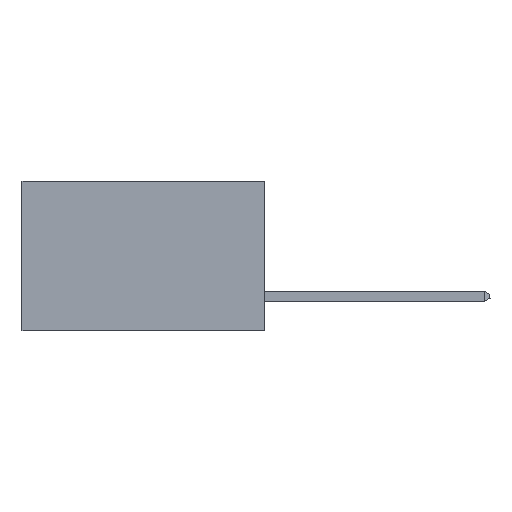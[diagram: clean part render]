
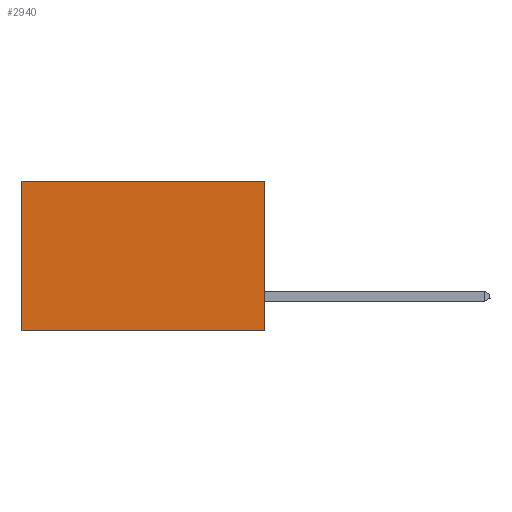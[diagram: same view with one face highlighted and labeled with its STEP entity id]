
A CAD part, left-side view. The second image highlights one B-rep face of the part: STEP entity #2940.
In plain terms, the highlighted planar face has unit normal (-1, 0, 0).
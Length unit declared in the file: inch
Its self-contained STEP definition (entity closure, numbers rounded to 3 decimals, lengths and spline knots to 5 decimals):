
#110 = VERTEX_POINT ( 'NONE', #6450 ) ;
#340 = DIRECTION ( 'NONE',  ( 0., 0., -1. ) ) ;
#413 = CARTESIAN_POINT ( 'NONE',  ( 0.298, 0., -0.37 ) ) ;
#958 = EDGE_CURVE ( 'NONE', #110, #6330, #5982, .T. ) ;
#1073 = EDGE_CURVE ( 'NONE', #6102, #6330, #7921, .T. ) ;
#1095 = EDGE_CURVE ( 'NONE', #4575, #6102, #7491, .T. ) ;
#1909 = CARTESIAN_POINT ( 'NONE',  ( 0.298, 0.6, 0. ) ) ;
#2111 = CARTESIAN_POINT ( 'NONE',  ( 0.298, 0., 0. ) ) ;
#2940 = ADVANCED_FACE ( 'NONE', ( #4148 ), #3633, .F. ) ;
#3633 = PLANE ( 'NONE',  #3737 ) ;
#3737 = AXIS2_PLACEMENT_3D ( 'NONE', #6610, #7228, #5591 ) ;
#3866 = CARTESIAN_POINT ( 'NONE',  ( 0.298, 0., -0.37 ) ) ;
#4030 = LINE ( 'NONE', #4324, #7432 ) ;
#4148 = FACE_OUTER_BOUND ( 'NONE', #8234, .T. ) ;
#4186 = VECTOR ( 'NONE', #8413, 39.37008 ) ;
#4272 = EDGE_CURVE ( 'NONE', #4575, #110, #4030, .T. ) ;
#4324 = CARTESIAN_POINT ( 'NONE',  ( 0.298, 0., 0. ) ) ;
#4575 = VERTEX_POINT ( 'NONE', #2111 ) ;
#5475 = VECTOR ( 'NONE', #340, 39.37008 ) ;
#5591 = DIRECTION ( 'NONE',  ( 0., 0., -1. ) ) ;
#5982 = LINE ( 'NONE', #1909, #4186 ) ;
#6102 = VERTEX_POINT ( 'NONE', #413 ) ;
#6123 = DIRECTION ( 'NONE',  ( 0., 1., 0. ) ) ;
#6330 = VERTEX_POINT ( 'NONE', #8139 ) ;
#6376 = ORIENTED_EDGE ( 'NONE', *, *, #1095, .F. ) ;
#6450 = CARTESIAN_POINT ( 'NONE',  ( 0.298, 0.6, 0. ) ) ;
#6549 = ORIENTED_EDGE ( 'NONE', *, *, #1073, .F. ) ;
#6610 = CARTESIAN_POINT ( 'NONE',  ( 0.298, 0., 0. ) ) ;
#6829 = ORIENTED_EDGE ( 'NONE', *, *, #958, .T. ) ;
#7228 = DIRECTION ( 'NONE',  ( 1., 0., 0. ) ) ;
#7432 = VECTOR ( 'NONE', #9420, 39.37008 ) ;
#7436 = ORIENTED_EDGE ( 'NONE', *, *, #4272, .T. ) ;
#7491 = LINE ( 'NONE', #7902, #5475 ) ;
#7902 = CARTESIAN_POINT ( 'NONE',  ( 0.298, 0., 0. ) ) ;
#7921 = LINE ( 'NONE', #3866, #9381 ) ;
#8139 = CARTESIAN_POINT ( 'NONE',  ( 0.298, 0.6, -0.37 ) ) ;
#8234 = EDGE_LOOP ( 'NONE', ( #6829, #6549, #6376, #7436 ) ) ;
#8413 = DIRECTION ( 'NONE',  ( 0., 0., -1. ) ) ;
#9381 = VECTOR ( 'NONE', #6123, 39.37008 ) ;
#9420 = DIRECTION ( 'NONE',  ( 0., 1., 0. ) ) ;
